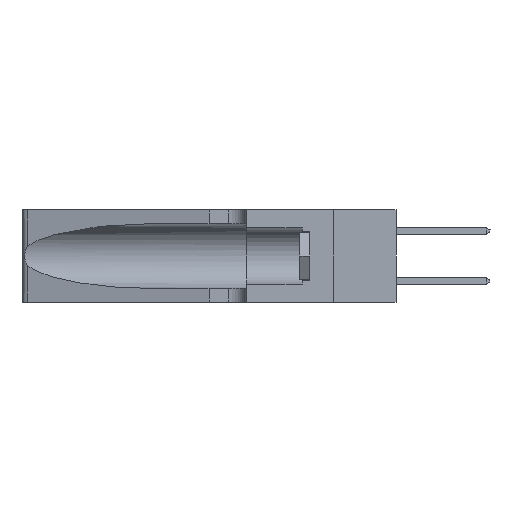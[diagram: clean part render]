
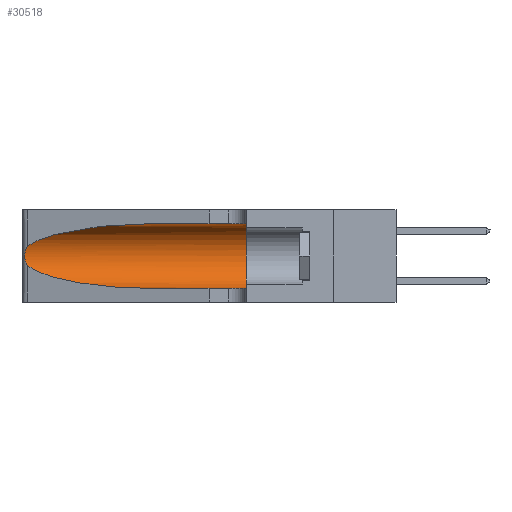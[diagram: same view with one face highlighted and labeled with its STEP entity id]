
A CAD part, left-side view. The second image highlights one B-rep face of the part: STEP entity #30518.
In plain terms, the highlighted cylindrical face has radius 3.308 mm (diameter 6.617 mm), a partial arc.
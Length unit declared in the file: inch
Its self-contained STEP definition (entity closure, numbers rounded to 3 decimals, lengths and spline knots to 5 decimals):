
#630 = CARTESIAN_POINT ( 'NONE',  ( 0.1305, 0.72297, 0.31525 ) ) ;
#719 = AXIS2_PLACEMENT_3D ( 'NONE', #33142, #21905, #36192 ) ;
#1473 = CARTESIAN_POINT ( 'NONE',  ( 0.1305, 0.35, 0.31525 ) ) ;
#1871 = CARTESIAN_POINT ( 'NONE',  ( 0.25555, 1.22993, 0.14849 ) ) ;
#2009 = CYLINDRICAL_SURFACE ( 'NONE', #4799, 0.13025 ) ;
#2261 = CARTESIAN_POINT ( 'NONE',  ( 0.25639, 1.23186, 0.15144 ) ) ;
#2876 = EDGE_CURVE ( 'NONE', #4072, #24942, #5688, .T. ) ;
#2984 = CARTESIAN_POINT ( 'NONE',  ( 0.25487, 1.22718, 0.14631 ) ) ;
#3076 = B_SPLINE_CURVE_WITH_KNOTS ( 'NONE', 3,
 ( #37228, #19499, #10684, #13638, #4941, #22552, #34051, #25348, #7844, #19361, #31337, #2261, #1871, #10925 ),
 .UNSPECIFIED., .F., .F.,
 ( 4, 2, 2, 2, 2, 2, 4 ),
 ( 0., 0.00027, 0.00053, 0.00107, 0.0016, 0.00187, 0.00214 ),
 .UNSPECIFIED. ) ;
#3455 = LINE ( 'NONE', #32785, #27634 ) ;
#4072 = VERTEX_POINT ( 'NONE', #1473 ) ;
#4799 = AXIS2_PLACEMENT_3D ( 'NONE', #20547, #11974, #6337 ) ;
#4941 = CARTESIAN_POINT ( 'NONE',  ( 0.25854, 1.2359, 0.20912 ) ) ;
#5688 = CIRCLE ( 'NONE', #719, 0.13025 ) ;
#6230 = CARTESIAN_POINT ( 'NONE',  ( 0.2373, 1.15595, 0.28018 ) ) ;
#6323 = EDGE_LOOP ( 'NONE', ( #30996, #26905, #6332, #36492, #15803, #25789 ) ) ;
#6332 = ORIENTED_EDGE ( 'NONE', *, *, #10341, .T. ) ;
#6337 = DIRECTION ( 'NONE',  ( 0., 0., -1. ) ) ;
#6756 = VERTEX_POINT ( 'NONE', #24770 ) ;
#7844 = CARTESIAN_POINT ( 'NONE',  ( 0.26017, 1.23833, 0.17102 ) ) ;
#8749 = EDGE_CURVE ( 'NONE', #20268, #4072, #15423, .T. ) ;
#8946 = CARTESIAN_POINT ( 'NONE',  ( 0.1305, 1.61858, 0.31525 ) ) ;
#10341 = EDGE_CURVE ( 'NONE', #18788, #34936, #11023, .T. ) ;
#10684 = CARTESIAN_POINT ( 'NONE',  ( 0.25639, 1.23184, 0.21858 ) ) ;
#10925 = CARTESIAN_POINT ( 'NONE',  ( 0.25487, 1.22718, 0.14631 ) ) ;
#11023 =( BOUNDED_CURVE ( )  B_SPLINE_CURVE ( 3, ( #28294, #25622, #19405, #37135 ),
 .UNSPECIFIED., .F., .T. ) 
 B_SPLINE_CURVE_WITH_KNOTS ( ( 4, 4 ),
 ( 3.44316, 4.71239 ),
 .UNSPECIFIED. ) 
 CURVE ( )  GEOMETRIC_REPRESENTATION_ITEM ( )  RATIONAL_B_SPLINE_CURVE ( ( 1., 0.87, 0.87, 1. ) ) 
 REPRESENTATION_ITEM ( '' )  );
#11491 =( BOUNDED_CURVE ( )  B_SPLINE_CURVE ( 3, ( #630, #23579, #6230, #20676 ),
 .UNSPECIFIED., .F., .T. ) 
 B_SPLINE_CURVE_WITH_KNOTS ( ( 4, 4 ),
 ( 1.5708, 2.84003 ),
 .UNSPECIFIED. ) 
 CURVE ( )  GEOMETRIC_REPRESENTATION_ITEM ( )  RATIONAL_B_SPLINE_CURVE ( ( 1., 0.87, 0.87, 1. ) ) 
 REPRESENTATION_ITEM ( '' )  );
#11974 = DIRECTION ( 'NONE',  ( 0., -1., 0. ) ) ;
#13638 = CARTESIAN_POINT ( 'NONE',  ( 0.25787, 1.23484, 0.2124 ) ) ;
#14130 = EDGE_CURVE ( 'NONE', #34936, #24942, #3455, .T. ) ;
#15423 = LINE ( 'NONE', #8946, #25863 ) ;
#15803 = ORIENTED_EDGE ( 'NONE', *, *, #2876, .F. ) ;
#16673 = CARTESIAN_POINT ( 'NONE',  ( 0.1305, 0.72297, 0.31525 ) ) ;
#18431 = FACE_OUTER_BOUND ( 'NONE', #6323, .T. ) ;
#18788 = VERTEX_POINT ( 'NONE', #2984 ) ;
#19361 = CARTESIAN_POINT ( 'NONE',  ( 0.25856, 1.23593, 0.16098 ) ) ;
#19405 = CARTESIAN_POINT ( 'NONE',  ( 0.18966, 0.96281, 0.05475 ) ) ;
#19499 = CARTESIAN_POINT ( 'NONE',  ( 0.25555, 1.22994, 0.2215 ) ) ;
#20268 = VERTEX_POINT ( 'NONE', #16673 ) ;
#20547 = CARTESIAN_POINT ( 'NONE',  ( 0.1305, 1.61858, 0.185 ) ) ;
#20676 = CARTESIAN_POINT ( 'NONE',  ( 0.25487, 1.22718, 0.22369 ) ) ;
#20805 = CARTESIAN_POINT ( 'NONE',  ( 0.1305, 0.35, 0.05475 ) ) ;
#20810 = DIRECTION ( 'NONE',  ( 0., -1., 0. ) ) ;
#21905 = DIRECTION ( 'NONE',  ( 0., 1., 0. ) ) ;
#22552 = CARTESIAN_POINT ( 'NONE',  ( 0.26018, 1.23835, 0.19895 ) ) ;
#23579 = CARTESIAN_POINT ( 'NONE',  ( 0.18966, 0.96281, 0.31525 ) ) ;
#24770 = CARTESIAN_POINT ( 'NONE',  ( 0.25487, 1.22718, 0.22369 ) ) ;
#24942 = VERTEX_POINT ( 'NONE', #20805 ) ;
#25348 = CARTESIAN_POINT ( 'NONE',  ( 0.26075, 1.23896, 0.178 ) ) ;
#25622 = CARTESIAN_POINT ( 'NONE',  ( 0.2373, 1.15595, 0.08982 ) ) ;
#25789 = ORIENTED_EDGE ( 'NONE', *, *, #8749, .F. ) ;
#25863 = VECTOR ( 'NONE', #37722, 39.37008 ) ;
#26905 = ORIENTED_EDGE ( 'NONE', *, *, #33108, .T. ) ;
#27634 = VECTOR ( 'NONE', #20810, 39.37008 ) ;
#28294 = CARTESIAN_POINT ( 'NONE',  ( 0.25487, 1.22718, 0.14631 ) ) ;
#28571 = EDGE_CURVE ( 'NONE', #20268, #6756, #11491, .T. ) ;
#30518 = ADVANCED_FACE ( 'NONE', ( #18431 ), #2009, .F. ) ;
#30996 = ORIENTED_EDGE ( 'NONE', *, *, #28571, .T. ) ;
#31337 = CARTESIAN_POINT ( 'NONE',  ( 0.25789, 1.23486, 0.15765 ) ) ;
#32785 = CARTESIAN_POINT ( 'NONE',  ( 0.1305, 1.61858, 0.05475 ) ) ;
#33108 = EDGE_CURVE ( 'NONE', #6756, #18788, #3076, .T. ) ;
#33142 = CARTESIAN_POINT ( 'NONE',  ( 0.1305, 0.35, 0.185 ) ) ;
#34051 = CARTESIAN_POINT ( 'NONE',  ( 0.26075, 1.23896, 0.19203 ) ) ;
#34936 = VERTEX_POINT ( 'NONE', #36110 ) ;
#36110 = CARTESIAN_POINT ( 'NONE',  ( 0.1305, 0.72297, 0.05475 ) ) ;
#36192 = DIRECTION ( 'NONE',  ( 0., 0., 1. ) ) ;
#36492 = ORIENTED_EDGE ( 'NONE', *, *, #14130, .T. ) ;
#37135 = CARTESIAN_POINT ( 'NONE',  ( 0.1305, 0.72297, 0.05475 ) ) ;
#37228 = CARTESIAN_POINT ( 'NONE',  ( 0.25487, 1.22718, 0.22369 ) ) ;
#37722 = DIRECTION ( 'NONE',  ( 0., -1., 0. ) ) ;
